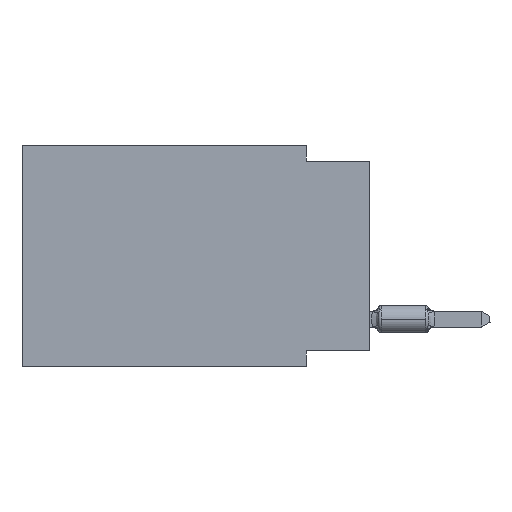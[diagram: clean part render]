
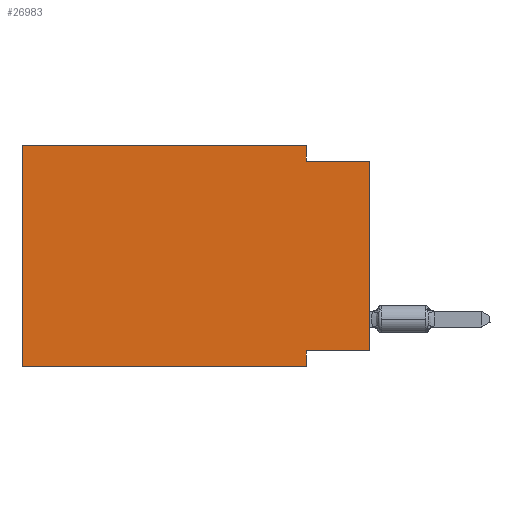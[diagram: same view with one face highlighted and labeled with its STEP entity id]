
A CAD part, left-side view. The second image highlights one B-rep face of the part: STEP entity #26983.
In plain terms, the highlighted planar face has unit normal (-1, 0, 0).
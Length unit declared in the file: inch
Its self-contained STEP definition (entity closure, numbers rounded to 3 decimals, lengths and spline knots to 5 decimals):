
#520 = LINE ( 'NONE', #14897, #47756 ) ;
#877 = DIRECTION ( 'NONE',  ( 0., 0., 1. ) ) ;
#1409 = CARTESIAN_POINT ( 'NONE',  ( 0., 0.55, -0.35 ) ) ;
#1556 = CARTESIAN_POINT ( 'NONE',  ( 0., 0.55, 0. ) ) ;
#2748 = CARTESIAN_POINT ( 'NONE',  ( 0., 0.55, 0. ) ) ;
#4656 = DIRECTION ( 'NONE',  ( 0., -1., 0. ) ) ;
#4763 = CARTESIAN_POINT ( 'NONE',  ( 0., 0., 0. ) ) ;
#6009 = LINE ( 'NONE', #1409, #34919 ) ;
#6156 = LINE ( 'NONE', #47282, #24564 ) ;
#8086 = DIRECTION ( 'NONE',  ( 0., 0., -1. ) ) ;
#8119 = ORIENTED_EDGE ( 'NONE', *, *, #18331, .F. ) ;
#8334 = DIRECTION ( 'NONE',  ( 1., 0., 0. ) ) ;
#10394 = ORIENTED_EDGE ( 'NONE', *, *, #29971, .F. ) ;
#10401 = EDGE_LOOP ( 'NONE', ( #26366, #10394, #26883, #8119, #33841, #26215, #27732, #34028 ) ) ;
#10443 = DIRECTION ( 'NONE',  ( 0., 0., -1. ) ) ;
#10580 = CARTESIAN_POINT ( 'NONE',  ( 0., 0., -0.325 ) ) ;
#11741 = FACE_OUTER_BOUND ( 'NONE', #10401, .T. ) ;
#14897 = CARTESIAN_POINT ( 'NONE',  ( 0., 0., -0.025 ) ) ;
#15809 = VERTEX_POINT ( 'NONE', #29070 ) ;
#16248 = DIRECTION ( 'NONE',  ( 0., -1., 0. ) ) ;
#16657 = VECTOR ( 'NONE', #10443, 39.37008 ) ;
#17438 = EDGE_CURVE ( 'NONE', #44537, #39404, #6156, .T. ) ;
#17951 = LINE ( 'NONE', #46421, #42361 ) ;
#18331 = EDGE_CURVE ( 'NONE', #30953, #15809, #32579, .T. ) ;
#20078 = VECTOR ( 'NONE', #877, 39.37008 ) ;
#20260 = LINE ( 'NONE', #1556, #43014 ) ;
#20343 = EDGE_CURVE ( 'NONE', #22865, #29477, #41753, .T. ) ;
#21097 = CARTESIAN_POINT ( 'NONE',  ( 0., 0.55, 0. ) ) ;
#21397 = CARTESIAN_POINT ( 'NONE',  ( 0., 0.1, -0.325 ) ) ;
#22865 = VERTEX_POINT ( 'NONE', #10580 ) ;
#23136 = CARTESIAN_POINT ( 'NONE',  ( 0., 0.55, -0.35 ) ) ;
#24564 = VECTOR ( 'NONE', #40472, 39.37008 ) ;
#26215 = ORIENTED_EDGE ( 'NONE', *, *, #38880, .T. ) ;
#26366 = ORIENTED_EDGE ( 'NONE', *, *, #20343, .T. ) ;
#26585 = PLANE ( 'NONE',  #46414 ) ;
#26883 = ORIENTED_EDGE ( 'NONE', *, *, #30091, .F. ) ;
#26983 = ADVANCED_FACE ( 'NONE', ( #11741 ), #26585, .F. ) ;
#27732 = ORIENTED_EDGE ( 'NONE', *, *, #17438, .F. ) ;
#27943 = DIRECTION ( 'NONE',  ( 0., 1., 0. ) ) ;
#29070 = CARTESIAN_POINT ( 'NONE',  ( 0., 0.1, 0. ) ) ;
#29477 = VERTEX_POINT ( 'NONE', #44619 ) ;
#29647 = EDGE_CURVE ( 'NONE', #29978, #30953, #20260, .T. ) ;
#29971 = EDGE_CURVE ( 'NONE', #42144, #29477, #520, .T. ) ;
#29978 = VERTEX_POINT ( 'NONE', #23136 ) ;
#30091 = EDGE_CURVE ( 'NONE', #15809, #42144, #33103, .T. ) ;
#30953 = VERTEX_POINT ( 'NONE', #2748 ) ;
#32579 = LINE ( 'NONE', #21097, #33965 ) ;
#32697 = EDGE_CURVE ( 'NONE', #22865, #44537, #17951, .T. ) ;
#33103 = LINE ( 'NONE', #40409, #16657 ) ;
#33665 = CARTESIAN_POINT ( 'NONE',  ( 0., 0.55, 0. ) ) ;
#33841 = ORIENTED_EDGE ( 'NONE', *, *, #29647, .F. ) ;
#33965 = VECTOR ( 'NONE', #43257, 39.37008 ) ;
#34028 = ORIENTED_EDGE ( 'NONE', *, *, #32697, .F. ) ;
#34919 = VECTOR ( 'NONE', #16248, 39.37008 ) ;
#38129 = CARTESIAN_POINT ( 'NONE',  ( 0., 0.1, -0.025 ) ) ;
#38880 = EDGE_CURVE ( 'NONE', #29978, #39404, #6009, .T. ) ;
#39404 = VERTEX_POINT ( 'NONE', #47563 ) ;
#40409 = CARTESIAN_POINT ( 'NONE',  ( 0., 0.1, 0. ) ) ;
#40472 = DIRECTION ( 'NONE',  ( 0., 0., -1. ) ) ;
#41753 = LINE ( 'NONE', #4763, #20078 ) ;
#42144 = VERTEX_POINT ( 'NONE', #38129 ) ;
#42361 = VECTOR ( 'NONE', #27943, 39.37008 ) ;
#42668 = DIRECTION ( 'NONE',  ( 0., 0., 1. ) ) ;
#43014 = VECTOR ( 'NONE', #42668, 39.37008 ) ;
#43257 = DIRECTION ( 'NONE',  ( 0., -1., 0. ) ) ;
#44537 = VERTEX_POINT ( 'NONE', #21397 ) ;
#44619 = CARTESIAN_POINT ( 'NONE',  ( 0., 0., -0.025 ) ) ;
#46414 = AXIS2_PLACEMENT_3D ( 'NONE', #33665, #8334, #8086 ) ;
#46421 = CARTESIAN_POINT ( 'NONE',  ( 0., 0., -0.325 ) ) ;
#47282 = CARTESIAN_POINT ( 'NONE',  ( 0., 0.1, -0.35 ) ) ;
#47563 = CARTESIAN_POINT ( 'NONE',  ( 0., 0.1, -0.35 ) ) ;
#47756 = VECTOR ( 'NONE', #4656, 39.37008 ) ;
